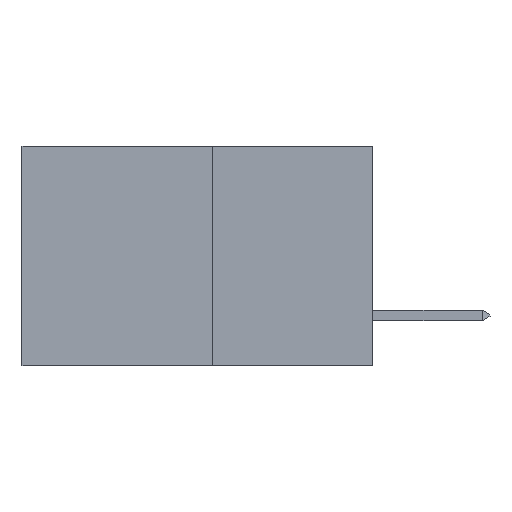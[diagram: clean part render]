
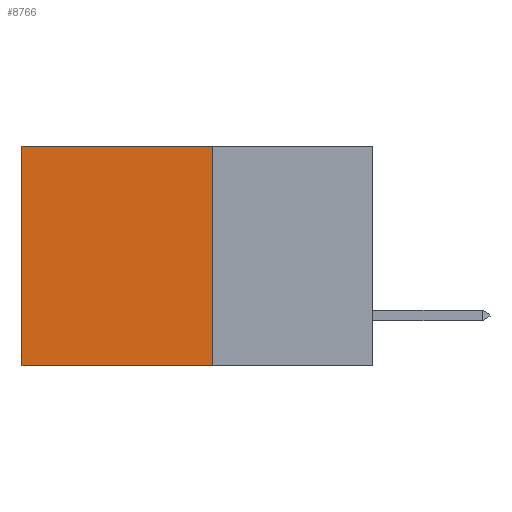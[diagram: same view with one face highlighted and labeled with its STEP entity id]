
A CAD part, left-side view. The second image highlights one B-rep face of the part: STEP entity #8766.
In plain terms, the highlighted planar face has unit normal (-1, 0, 0).
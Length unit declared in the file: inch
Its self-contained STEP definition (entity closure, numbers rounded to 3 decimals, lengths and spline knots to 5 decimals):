
#730 = ORIENTED_EDGE ( 'NONE', *, *, #1105, .T. ) ;
#734 = ORIENTED_EDGE ( 'NONE', *, *, #834, .F. ) ;
#834 = EDGE_CURVE ( 'NONE', #5735, #9015, #1369, .T. ) ;
#1105 = EDGE_CURVE ( 'NONE', #1180, #10047, #1215, .T. ) ;
#1180 = VERTEX_POINT ( 'NONE', #7025 ) ;
#1200 = DIRECTION ( 'NONE',  ( 0., 1., 0. ) ) ;
#1215 = LINE ( 'NONE', #5854, #3623 ) ;
#1255 = LINE ( 'NONE', #10874, #10957 ) ;
#1369 = LINE ( 'NONE', #6529, #8552 ) ;
#1578 = CARTESIAN_POINT ( 'NONE',  ( 0.277, 0.27, -0.37 ) ) ;
#2918 = CARTESIAN_POINT ( 'NONE',  ( 0.277, 0.59, -0.37 ) ) ;
#3623 = VECTOR ( 'NONE', #1200, 39.37008 ) ;
#3983 = CARTESIAN_POINT ( 'NONE',  ( 0.277, 0.59, 0. ) ) ;
#4450 = DIRECTION ( 'NONE',  ( 0., 0., -1. ) ) ;
#4604 = EDGE_CURVE ( 'NONE', #10047, #9015, #1255, .T. ) ;
#5192 = CARTESIAN_POINT ( 'NONE',  ( 0.277, 0.27, -0.37 ) ) ;
#5735 = VERTEX_POINT ( 'NONE', #1578 ) ;
#5854 = CARTESIAN_POINT ( 'NONE',  ( 0.277, 0.27, 0. ) ) ;
#5901 = FACE_OUTER_BOUND ( 'NONE', #7577, .T. ) ;
#5953 = AXIS2_PLACEMENT_3D ( 'NONE', #6326, #10112, #4450 ) ;
#6326 = CARTESIAN_POINT ( 'NONE',  ( 0.277, 0.27, -0.37 ) ) ;
#6529 = CARTESIAN_POINT ( 'NONE',  ( 0.277, 0.27, -0.37 ) ) ;
#6727 = DIRECTION ( 'NONE',  ( 0., 1., 0. ) ) ;
#7025 = CARTESIAN_POINT ( 'NONE',  ( 0.277, 0.27, 0. ) ) ;
#7137 = DIRECTION ( 'NONE',  ( 0., 0., -1. ) ) ;
#7201 = VECTOR ( 'NONE', #7137, 39.37008 ) ;
#7577 = EDGE_LOOP ( 'NONE', ( #8130, #734, #9764, #730 ) ) ;
#8130 = ORIENTED_EDGE ( 'NONE', *, *, #4604, .T. ) ;
#8219 = PLANE ( 'NONE',  #5953 ) ;
#8552 = VECTOR ( 'NONE', #6727, 39.37008 ) ;
#8766 = ADVANCED_FACE ( 'NONE', ( #5901 ), #8219, .F. ) ;
#9015 = VERTEX_POINT ( 'NONE', #2918 ) ;
#9674 = LINE ( 'NONE', #5192, #7201 ) ;
#9764 = ORIENTED_EDGE ( 'NONE', *, *, #11052, .F. ) ;
#10047 = VERTEX_POINT ( 'NONE', #3983 ) ;
#10112 = DIRECTION ( 'NONE',  ( 1., 0., 0. ) ) ;
#10874 = CARTESIAN_POINT ( 'NONE',  ( 0.277, 0.59, -0.37 ) ) ;
#10898 = DIRECTION ( 'NONE',  ( 0., 0., -1. ) ) ;
#10957 = VECTOR ( 'NONE', #10898, 39.37008 ) ;
#11052 = EDGE_CURVE ( 'NONE', #1180, #5735, #9674, .T. ) ;
